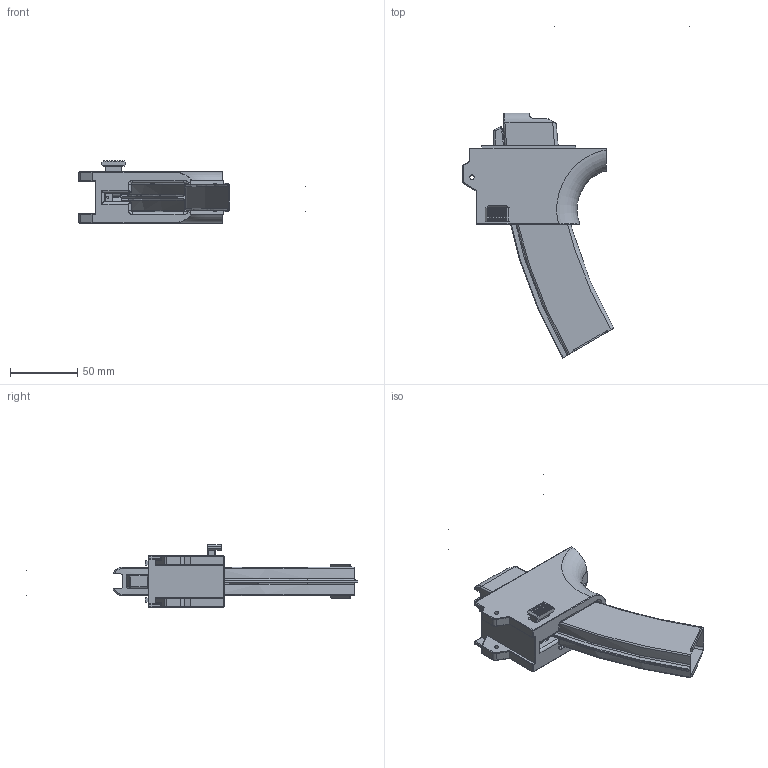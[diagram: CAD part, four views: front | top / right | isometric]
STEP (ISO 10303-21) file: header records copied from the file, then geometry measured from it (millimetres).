
FILE_DESCRIPTION(/* description */ (''),/* implementation_level */ '2;1');
FILE_NAME(/* name */ 'MOD9 PPS43 MAGWELL.stp',/* time_stamp */ '2021-07-08T22:19:12+02:00',/* author */ (''),/* organization */ (''),/* preprocessor_version */ 'ST-DEVELOPER v15.2',/* originating_system */ 'Autodesk Translator Framework v2.0.0.5431',/* authorisation */ '');
FILE_SCHEMA (('AUTOMOTIVE_DESIGN { 1 0 10303 214 3 1 1 }'));
Length unit declared in the file: centimetre
Products named in the file (1): PPS43 MAGWELL MOD9 FINAL V3
Bounding box: 168.26 x 246.42 x 46.13 mm (x, y, z)
Volume: 140716.2 mm3; surface area: 74488.4 mm2
Topology: 8 solids, 8 shells, 851 faces, 2219 edges, 1389 vertices
Faces by surface type: bspline 367, plane 248, cylinder 162, torus 38, cone 20, sphere 16
Full cylindrical faces by diameter (mm): 1.3 x1, 1.4 x1, 1.6 x1, 3.4 x2, 4 x2
Entity records: 31956 total; most frequent: CARTESIAN_POINT 13273, ORIENTED_EDGE 4406, DIRECTION 2969, EDGE_CURVE 2203, VERTEX_POINT 1389, LINE 1001, VECTOR 1001, AXIS2_PLACEMENT_3D 984
